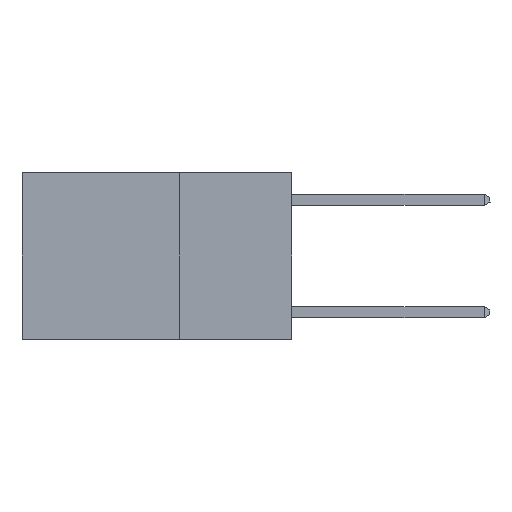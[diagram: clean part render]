
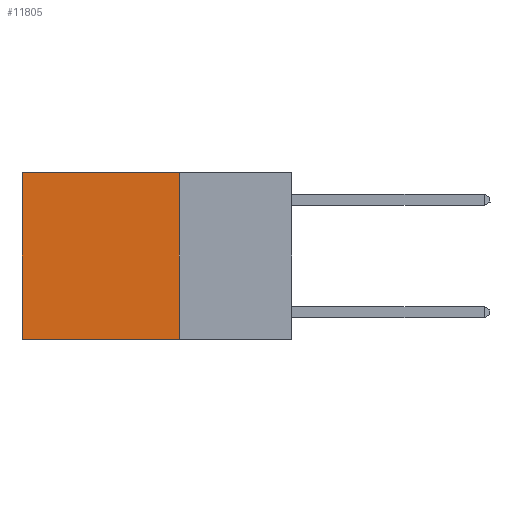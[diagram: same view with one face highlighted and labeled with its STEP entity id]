
A CAD part, left-side view. The second image highlights one B-rep face of the part: STEP entity #11805.
In plain terms, the highlighted planar face has unit normal (-1, 0, 0).
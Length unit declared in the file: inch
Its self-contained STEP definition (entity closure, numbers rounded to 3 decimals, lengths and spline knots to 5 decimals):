
#608 = ORIENTED_EDGE ( 'NONE', *, *, #13455, .F. ) ;
#1915 = CARTESIAN_POINT ( 'NONE',  ( 0.2625, 0.25, 0. ) ) ;
#2429 = VERTEX_POINT ( 'NONE', #7988 ) ;
#3635 = LINE ( 'NONE', #5549, #18454 ) ;
#5456 = EDGE_CURVE ( 'NONE', #10958, #2429, #3635, .T. ) ;
#5549 = CARTESIAN_POINT ( 'NONE',  ( 0.2625, 0.25, 0. ) ) ;
#7761 = CARTESIAN_POINT ( 'NONE',  ( 0.2625, 0.6, -0.37 ) ) ;
#7905 = ORIENTED_EDGE ( 'NONE', *, *, #14639, .F. ) ;
#7988 = CARTESIAN_POINT ( 'NONE',  ( 0.2625, 0.6, 0. ) ) ;
#8946 = EDGE_LOOP ( 'NONE', ( #19236, #608, #7905, #21461 ) ) ;
#9709 = DIRECTION ( 'NONE',  ( 0., 1., 0. ) ) ;
#10719 = PLANE ( 'NONE',  #16871 ) ;
#10958 = VERTEX_POINT ( 'NONE', #1915 ) ;
#11503 = FACE_OUTER_BOUND ( 'NONE', #8946, .T. ) ;
#11805 = ADVANCED_FACE ( 'NONE', ( #11503 ), #10719, .F. ) ;
#12824 = DIRECTION ( 'NONE',  ( 0., 0., -1. ) ) ;
#13455 = EDGE_CURVE ( 'NONE', #14687, #17610, #19351, .T. ) ;
#14024 = DIRECTION ( 'NONE',  ( 0., 1., 0. ) ) ;
#14597 = DIRECTION ( 'NONE',  ( 0., 0., -1. ) ) ;
#14639 = EDGE_CURVE ( 'NONE', #10958, #14687, #19281, .T. ) ;
#14687 = VERTEX_POINT ( 'NONE', #16853 ) ;
#14981 = DIRECTION ( 'NONE',  ( 0., 0., -1. ) ) ;
#16212 = VECTOR ( 'NONE', #14597, 39.37008 ) ;
#16853 = CARTESIAN_POINT ( 'NONE',  ( 0.2625, 0.25, -0.37 ) ) ;
#16871 = AXIS2_PLACEMENT_3D ( 'NONE', #22441, #24617, #12824 ) ;
#17055 = CARTESIAN_POINT ( 'NONE',  ( 0.2625, 0.25, 0. ) ) ;
#17610 = VERTEX_POINT ( 'NONE', #7761 ) ;
#18454 = VECTOR ( 'NONE', #9709, 39.37008 ) ;
#18849 = VECTOR ( 'NONE', #14981, 39.37008 ) ;
#19236 = ORIENTED_EDGE ( 'NONE', *, *, #22042, .T. ) ;
#19281 = LINE ( 'NONE', #17055, #16212 ) ;
#19351 = LINE ( 'NONE', #19799, #23286 ) ;
#19799 = CARTESIAN_POINT ( 'NONE',  ( 0.2625, 0.25, -0.37 ) ) ;
#20909 = CARTESIAN_POINT ( 'NONE',  ( 0.2625, 0.6, 0. ) ) ;
#21461 = ORIENTED_EDGE ( 'NONE', *, *, #5456, .T. ) ;
#22042 = EDGE_CURVE ( 'NONE', #2429, #17610, #23971, .T. ) ;
#22441 = CARTESIAN_POINT ( 'NONE',  ( 0.2625, 0.25, 0. ) ) ;
#23286 = VECTOR ( 'NONE', #14024, 39.37008 ) ;
#23971 = LINE ( 'NONE', #20909, #18849 ) ;
#24617 = DIRECTION ( 'NONE',  ( 1., 0., 0. ) ) ;
